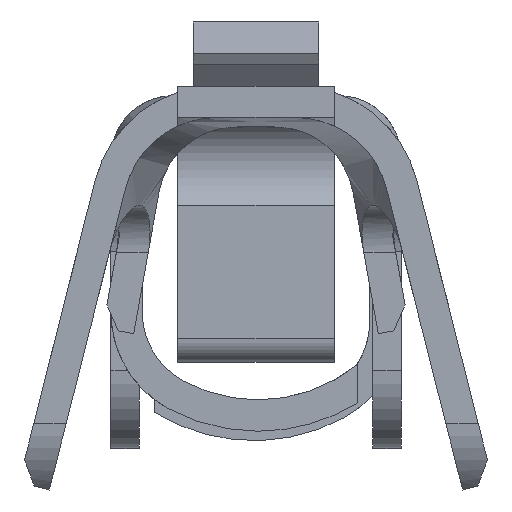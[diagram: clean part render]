
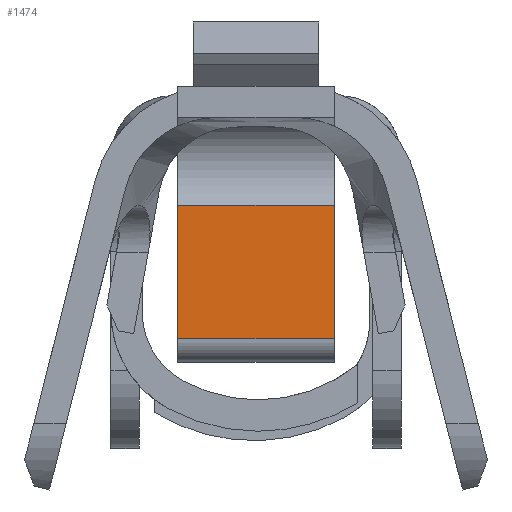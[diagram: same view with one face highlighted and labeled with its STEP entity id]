
A CAD part, front view. The second image highlights one B-rep face of the part: STEP entity #1474.
In plain terms, the highlighted planar face has unit normal (0, -1, 0).
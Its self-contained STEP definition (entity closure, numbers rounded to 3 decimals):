
#1 = LINE ( 'NONE', #4253, #380 ) ;
#48 = DIRECTION ( 'NONE',  ( -1., 0., 0. ) ) ;
#133 = PLANE ( 'NONE',  #2642 ) ;
#380 = VECTOR ( 'NONE', #48, 1000. ) ;
#503 = CARTESIAN_POINT ( 'NONE',  ( 0.5, 4.2, -1.61 ) ) ;
#544 = EDGE_CURVE ( 'NONE', #3359, #3347, #2540, .T. ) ;
#630 = DIRECTION ( 'NONE',  ( 0., 0., -1. ) ) ;
#759 = LINE ( 'NONE', #2085, #3217 ) ;
#801 = ORIENTED_EDGE ( 'NONE', *, *, #544, .T. ) ;
#871 = DIRECTION ( 'NONE',  ( 0., 0., -1. ) ) ;
#1474 = ADVANCED_FACE ( 'NONE', ( #2117 ), #133, .F. ) ;
#1705 = ORIENTED_EDGE ( 'NONE', *, *, #3642, .F. ) ;
#1748 = VERTEX_POINT ( 'NONE', #2287 ) ;
#1839 = ORIENTED_EDGE ( 'NONE', *, *, #1860, .F. ) ;
#1860 = EDGE_CURVE ( 'NONE', #3272, #1748, #3806, .T. ) ;
#2073 = DIRECTION ( 'NONE',  ( 0., 0., 1. ) ) ;
#2085 = CARTESIAN_POINT ( 'NONE',  ( 0.5, 4.2, -0.76 ) ) ;
#2117 = FACE_OUTER_BOUND ( 'NONE', #3944, .T. ) ;
#2287 = CARTESIAN_POINT ( 'NONE',  ( 0.5, 4.2, -1.61 ) ) ;
#2502 = VECTOR ( 'NONE', #871, 1000. ) ;
#2515 = CARTESIAN_POINT ( 'NONE',  ( -0.5, 4.2, -0.76 ) ) ;
#2540 = LINE ( 'NONE', #4196, #2777 ) ;
#2642 = AXIS2_PLACEMENT_3D ( 'NONE', #4063, #2767, #2073 ) ;
#2722 = ORIENTED_EDGE ( 'NONE', *, *, #3275, .T. ) ;
#2767 = DIRECTION ( 'NONE',  ( 0., 1., 0. ) ) ;
#2777 = VECTOR ( 'NONE', #630, 1000. ) ;
#3217 = VECTOR ( 'NONE', #3418, 1000. ) ;
#3272 = VERTEX_POINT ( 'NONE', #3742 ) ;
#3275 = EDGE_CURVE ( 'NONE', #3272, #3359, #759, .T. ) ;
#3347 = VERTEX_POINT ( 'NONE', #3542 ) ;
#3359 = VERTEX_POINT ( 'NONE', #2515 ) ;
#3418 = DIRECTION ( 'NONE',  ( -1., 0., 0. ) ) ;
#3542 = CARTESIAN_POINT ( 'NONE',  ( -0.5, 4.2, -1.61 ) ) ;
#3642 = EDGE_CURVE ( 'NONE', #1748, #3347, #1, .T. ) ;
#3742 = CARTESIAN_POINT ( 'NONE',  ( 0.5, 4.2, -0.76 ) ) ;
#3806 = LINE ( 'NONE', #503, #2502 ) ;
#3944 = EDGE_LOOP ( 'NONE', ( #801, #1705, #1839, #2722 ) ) ;
#4063 = CARTESIAN_POINT ( 'NONE',  ( 0.5, 4.2, -1.61 ) ) ;
#4196 = CARTESIAN_POINT ( 'NONE',  ( -0.5, 4.2, -1.61 ) ) ;
#4253 = CARTESIAN_POINT ( 'NONE',  ( 0.5, 4.2, -1.61 ) ) ;
